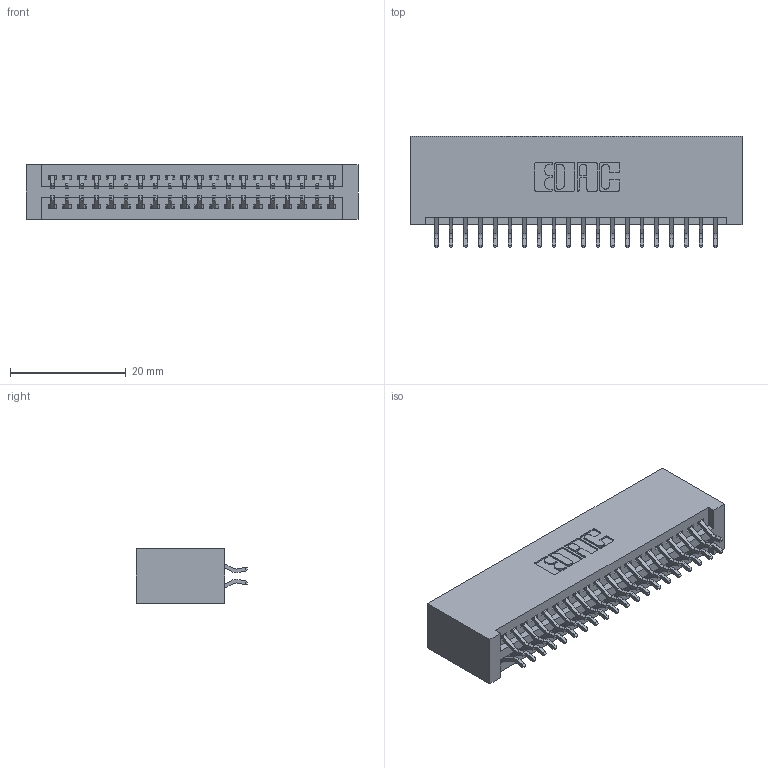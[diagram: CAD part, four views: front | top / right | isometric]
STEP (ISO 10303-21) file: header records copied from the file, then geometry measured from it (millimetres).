
FILE_DESCRIPTION (( 'STEP AP203' ), '1' );
FILE_NAME ('345-040-556-201.STEP', '2019-10-28T18:14:11', ( '' ), ( '' ), 'SwSTEP 2.0', 'SolidWorks 2016', '' );
FILE_SCHEMA (( 'CONFIG_CONTROL_DESIGN' ));
Length unit declared in the file: inch
Products named in the file (3): 345-040-556-201; 345 Part_No Mounting Lugs; 345-292-001_556 Tail
Assembly tree (41 placements, depth 2):
  345-040-556-201
    345 Part_No Mounting Lugs
    345-292-001_556 Tail  x40
Bounding box: 57.4 x 19.24 x 9.4 mm (x, y, z)
Volume: 5986.4 mm3; surface area: 8691.1 mm2
Topology: 41 solids, 41 shells, 2358 faces, 6997 edges, 4610 vertices
Faces by surface type: plane 1556, cylinder 802
Entity records: 18597 total; most frequent: CARTESIAN_POINT 3152, ORIENTED_EDGE 3074, DIRECTION 2789, EDGE_CURVE 1537, VECTOR 1325, LINE 1325, VERTEX_POINT 1022, AXIS2_PLACEMENT_3D 732
